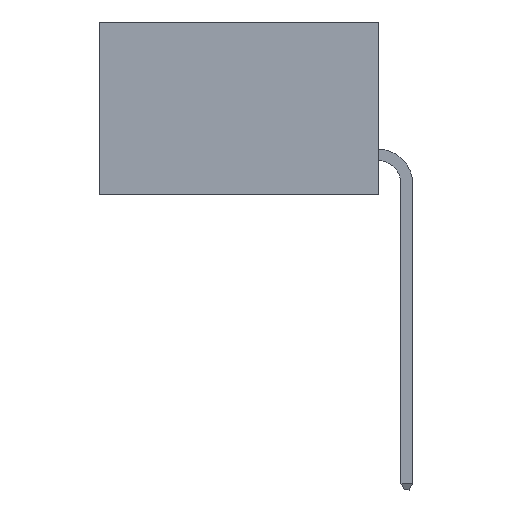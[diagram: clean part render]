
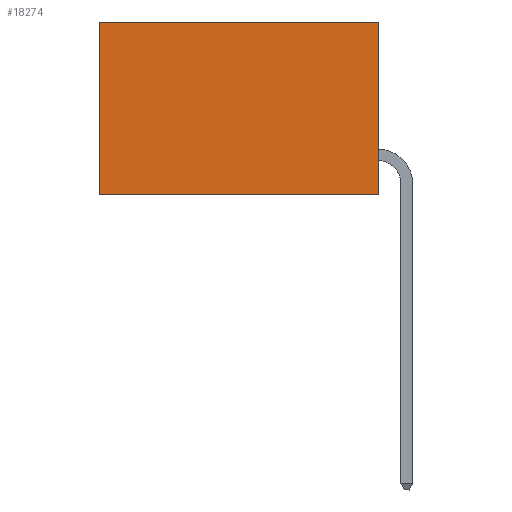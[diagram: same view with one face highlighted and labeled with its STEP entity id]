
A CAD part, left-side view. The second image highlights one B-rep face of the part: STEP entity #18274.
In plain terms, the highlighted planar face has unit normal (-1, 0, 0).
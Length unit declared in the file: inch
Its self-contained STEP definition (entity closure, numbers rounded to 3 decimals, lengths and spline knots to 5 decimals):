
#2342 = EDGE_CURVE ( 'NONE', #24630, #9241, #26578, .T. ) ;
#2636 = PLANE ( 'NONE',  #6437 ) ;
#3435 = CARTESIAN_POINT ( 'NONE',  ( 0.298, 0., 0. ) ) ;
#4408 = VERTEX_POINT ( 'NONE', #4478 ) ;
#4478 = CARTESIAN_POINT ( 'NONE',  ( 0.298, 0.6, 0. ) ) ;
#4822 = ORIENTED_EDGE ( 'NONE', *, *, #22471, .F. ) ;
#5078 = LINE ( 'NONE', #23494, #20305 ) ;
#6437 = AXIS2_PLACEMENT_3D ( 'NONE', #6740, #21271, #8846 ) ;
#6696 = CARTESIAN_POINT ( 'NONE',  ( 0.298, 0., -0.37 ) ) ;
#6740 = CARTESIAN_POINT ( 'NONE',  ( 0.298, 0., 0. ) ) ;
#8264 = ORIENTED_EDGE ( 'NONE', *, *, #22230, .T. ) ;
#8846 = DIRECTION ( 'NONE',  ( 0., 0., -1. ) ) ;
#9241 = VERTEX_POINT ( 'NONE', #9258 ) ;
#9258 = CARTESIAN_POINT ( 'NONE',  ( 0.298, 0., -0.37 ) ) ;
#9607 = ORIENTED_EDGE ( 'NONE', *, *, #22916, .T. ) ;
#10114 = VECTOR ( 'NONE', #16685, 39.37008 ) ;
#10363 = CARTESIAN_POINT ( 'NONE',  ( 0.298, 0.6, 0. ) ) ;
#10922 = DIRECTION ( 'NONE',  ( 0., 1., 0. ) ) ;
#12850 = EDGE_LOOP ( 'NONE', ( #9607, #4822, #19844, #8264 ) ) ;
#13056 = VERTEX_POINT ( 'NONE', #23052 ) ;
#13139 = FACE_OUTER_BOUND ( 'NONE', #12850, .T. ) ;
#15104 = LINE ( 'NONE', #6696, #25460 ) ;
#15707 = VECTOR ( 'NONE', #16579, 39.37008 ) ;
#16579 = DIRECTION ( 'NONE',  ( 0., 0., -1. ) ) ;
#16685 = DIRECTION ( 'NONE',  ( 0., 0., -1. ) ) ;
#18274 = ADVANCED_FACE ( 'NONE', ( #13139 ), #2636, .F. ) ;
#19844 = ORIENTED_EDGE ( 'NONE', *, *, #2342, .F. ) ;
#20305 = VECTOR ( 'NONE', #21492, 39.37008 ) ;
#21193 = LINE ( 'NONE', #10363, #15707 ) ;
#21271 = DIRECTION ( 'NONE',  ( 1., 0., 0. ) ) ;
#21492 = DIRECTION ( 'NONE',  ( 0., 1., 0. ) ) ;
#22205 = CARTESIAN_POINT ( 'NONE',  ( 0.298, 0., 0. ) ) ;
#22230 = EDGE_CURVE ( 'NONE', #24630, #4408, #5078, .T. ) ;
#22471 = EDGE_CURVE ( 'NONE', #9241, #13056, #15104, .T. ) ;
#22916 = EDGE_CURVE ( 'NONE', #4408, #13056, #21193, .T. ) ;
#23052 = CARTESIAN_POINT ( 'NONE',  ( 0.298, 0.6, -0.37 ) ) ;
#23494 = CARTESIAN_POINT ( 'NONE',  ( 0.298, 0., 0. ) ) ;
#24630 = VERTEX_POINT ( 'NONE', #22205 ) ;
#25460 = VECTOR ( 'NONE', #10922, 39.37008 ) ;
#26578 = LINE ( 'NONE', #3435, #10114 ) ;
